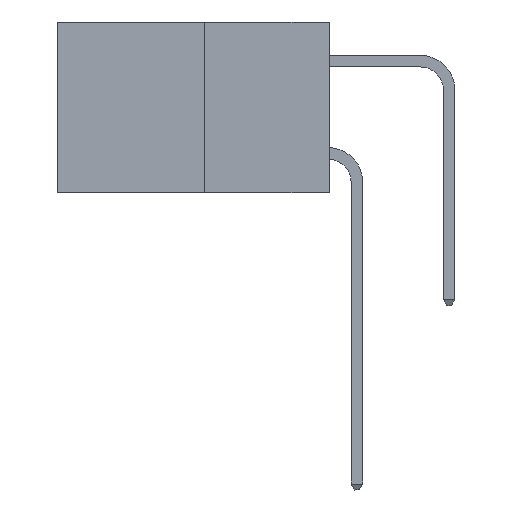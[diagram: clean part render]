
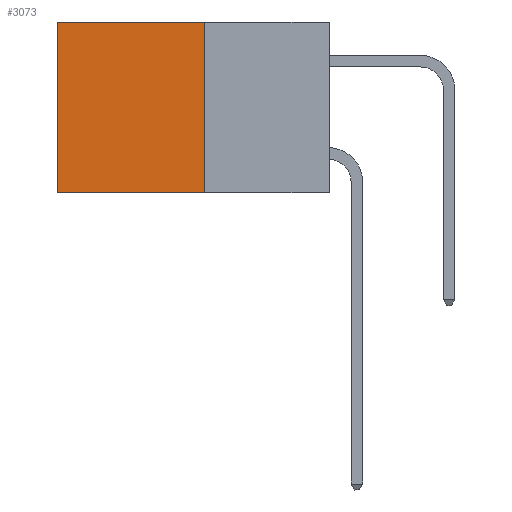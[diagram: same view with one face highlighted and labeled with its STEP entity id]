
A CAD part, left-side view. The second image highlights one B-rep face of the part: STEP entity #3073.
In plain terms, the highlighted planar face has unit normal (-1, 0, 0).
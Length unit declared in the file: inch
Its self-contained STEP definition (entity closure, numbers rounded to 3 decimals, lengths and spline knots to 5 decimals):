
#113 = VERTEX_POINT ( 'NONE', #11020 ) ;
#242 = EDGE_CURVE ( 'NONE', #5901, #113, #10848, .T. ) ;
#1030 = CARTESIAN_POINT ( 'NONE',  ( 0.277, 0.27, -0.37 ) ) ;
#1123 = EDGE_CURVE ( 'NONE', #3226, #5901, #4712, .T. ) ;
#1236 = DIRECTION ( 'NONE',  ( 0., 1., 0. ) ) ;
#1736 = VECTOR ( 'NONE', #11315, 39.37008 ) ;
#1797 = CARTESIAN_POINT ( 'NONE',  ( 0.277, 0.59, -0.37 ) ) ;
#2765 = DIRECTION ( 'NONE',  ( 0., 0., -1. ) ) ;
#2971 = CARTESIAN_POINT ( 'NONE',  ( 0.277, 0.27, 0. ) ) ;
#3073 = ADVANCED_FACE ( 'NONE', ( #4692 ), #7762, .F. ) ;
#3226 = VERTEX_POINT ( 'NONE', #2971 ) ;
#3984 = VECTOR ( 'NONE', #1236, 39.37008 ) ;
#4193 = CARTESIAN_POINT ( 'NONE',  ( 0.277, 0.59, 0. ) ) ;
#4412 = VECTOR ( 'NONE', #11263, 39.37008 ) ;
#4692 = FACE_OUTER_BOUND ( 'NONE', #7652, .T. ) ;
#4712 = LINE ( 'NONE', #8715, #4412 ) ;
#4849 = EDGE_CURVE ( 'NONE', #3226, #11137, #8860, .T. ) ;
#5472 = DIRECTION ( 'NONE',  ( 0., 0., -1. ) ) ;
#5901 = VERTEX_POINT ( 'NONE', #9653 ) ;
#5990 = DIRECTION ( 'NONE',  ( 1., 0., 0. ) ) ;
#6481 = CARTESIAN_POINT ( 'NONE',  ( 0.277, 0.27, -0.37 ) ) ;
#6963 = ORIENTED_EDGE ( 'NONE', *, *, #10386, .T. ) ;
#7019 = ORIENTED_EDGE ( 'NONE', *, *, #242, .F. ) ;
#7180 = ORIENTED_EDGE ( 'NONE', *, *, #1123, .F. ) ;
#7363 = ORIENTED_EDGE ( 'NONE', *, *, #4849, .T. ) ;
#7652 = EDGE_LOOP ( 'NONE', ( #6963, #7019, #7180, #7363 ) ) ;
#7755 = AXIS2_PLACEMENT_3D ( 'NONE', #6481, #5990, #5472 ) ;
#7762 = PLANE ( 'NONE',  #7755 ) ;
#8538 = VECTOR ( 'NONE', #2765, 39.37008 ) ;
#8715 = CARTESIAN_POINT ( 'NONE',  ( 0.277, 0.27, -0.37 ) ) ;
#8773 = CARTESIAN_POINT ( 'NONE',  ( 0.277, 0.27, 0. ) ) ;
#8860 = LINE ( 'NONE', #8773, #1736 ) ;
#9653 = CARTESIAN_POINT ( 'NONE',  ( 0.277, 0.27, -0.37 ) ) ;
#10386 = EDGE_CURVE ( 'NONE', #11137, #113, #10823, .T. ) ;
#10823 = LINE ( 'NONE', #1797, #8538 ) ;
#10848 = LINE ( 'NONE', #1030, #3984 ) ;
#11020 = CARTESIAN_POINT ( 'NONE',  ( 0.277, 0.59, -0.37 ) ) ;
#11137 = VERTEX_POINT ( 'NONE', #4193 ) ;
#11263 = DIRECTION ( 'NONE',  ( 0., 0., -1. ) ) ;
#11315 = DIRECTION ( 'NONE',  ( 0., 1., 0. ) ) ;
